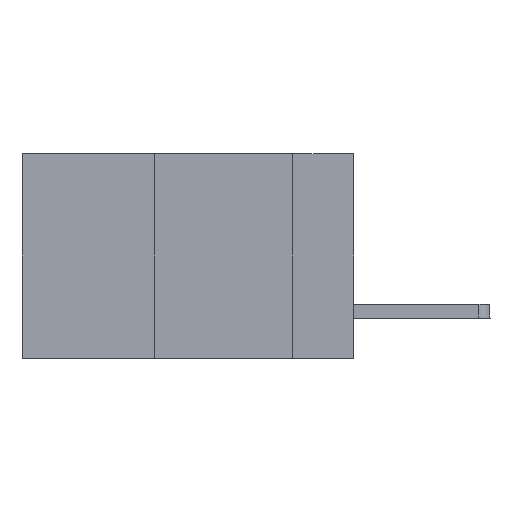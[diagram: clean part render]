
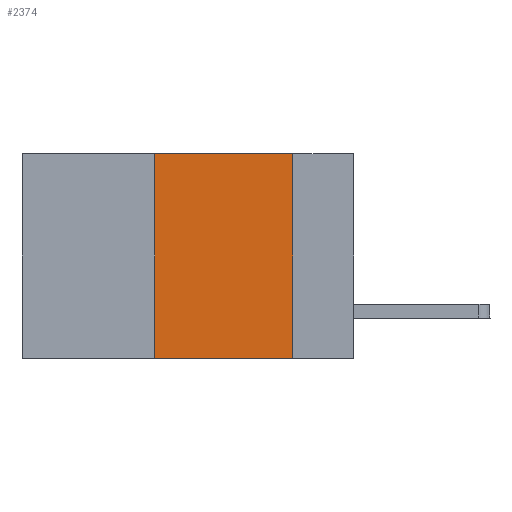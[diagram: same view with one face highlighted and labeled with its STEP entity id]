
A CAD part, left-side view. The second image highlights one B-rep face of the part: STEP entity #2374.
In plain terms, the highlighted planar face has unit normal (-1, 0, 0).
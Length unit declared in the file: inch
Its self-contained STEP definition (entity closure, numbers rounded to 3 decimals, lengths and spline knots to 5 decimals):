
#46 = EDGE_CURVE ( 'NONE', #2025, #4561, #7587, .T. ) ;
#168 = LINE ( 'NONE', #4430, #11557 ) ;
#1064 = VERTEX_POINT ( 'NONE', #3445 ) ;
#1229 = VERTEX_POINT ( 'NONE', #8865 ) ;
#1860 = CARTESIAN_POINT ( 'NONE',  ( 0., 0.11, 0. ) ) ;
#2025 = VERTEX_POINT ( 'NONE', #5776 ) ;
#2374 = ADVANCED_FACE ( 'NONE', ( #10381 ), #6928, .F. ) ;
#2579 = ORIENTED_EDGE ( 'NONE', *, *, #8840, .F. ) ;
#2673 = VECTOR ( 'NONE', #3794, 39.37008 ) ;
#2675 = VECTOR ( 'NONE', #6102, 39.37008 ) ;
#3445 = CARTESIAN_POINT ( 'NONE',  ( 0., 0.11, -0.37 ) ) ;
#3711 = EDGE_CURVE ( 'NONE', #1229, #2025, #168, .T. ) ;
#3794 = DIRECTION ( 'NONE',  ( 0., 0., -1. ) ) ;
#4235 = DIRECTION ( 'NONE',  ( 0., 0., -1. ) ) ;
#4430 = CARTESIAN_POINT ( 'NONE',  ( 0., 0.36, 0. ) ) ;
#4561 = VERTEX_POINT ( 'NONE', #9695 ) ;
#5181 = LINE ( 'NONE', #1860, #2673 ) ;
#5776 = CARTESIAN_POINT ( 'NONE',  ( 0., 0.36, 0. ) ) ;
#6102 = DIRECTION ( 'NONE',  ( 0., -1., 0. ) ) ;
#6368 = DIRECTION ( 'NONE',  ( 0., 0., 1. ) ) ;
#6550 = DIRECTION ( 'NONE',  ( 0., -1., 0. ) ) ;
#6928 = PLANE ( 'NONE',  #7059 ) ;
#7059 = AXIS2_PLACEMENT_3D ( 'NONE', #9151, #8613, #4235 ) ;
#7584 = VECTOR ( 'NONE', #6550, 39.37008 ) ;
#7587 = LINE ( 'NONE', #11451, #2675 ) ;
#8382 = ORIENTED_EDGE ( 'NONE', *, *, #46, .F. ) ;
#8613 = DIRECTION ( 'NONE',  ( 1., 0., 0. ) ) ;
#8840 = EDGE_CURVE ( 'NONE', #4561, #1064, #5181, .T. ) ;
#8855 = EDGE_CURVE ( 'NONE', #1229, #1064, #10034, .T. ) ;
#8865 = CARTESIAN_POINT ( 'NONE',  ( 0., 0.36, -0.37 ) ) ;
#8937 = ORIENTED_EDGE ( 'NONE', *, *, #3711, .F. ) ;
#9151 = CARTESIAN_POINT ( 'NONE',  ( 0., 0.6, 0. ) ) ;
#9695 = CARTESIAN_POINT ( 'NONE',  ( 0., 0.11, 0. ) ) ;
#10034 = LINE ( 'NONE', #10169, #7584 ) ;
#10169 = CARTESIAN_POINT ( 'NONE',  ( 0., 0.6, -0.37 ) ) ;
#10301 = EDGE_LOOP ( 'NONE', ( #2579, #8382, #8937, #11395 ) ) ;
#10381 = FACE_OUTER_BOUND ( 'NONE', #10301, .T. ) ;
#11395 = ORIENTED_EDGE ( 'NONE', *, *, #8855, .T. ) ;
#11451 = CARTESIAN_POINT ( 'NONE',  ( 0., 0.6, 0. ) ) ;
#11557 = VECTOR ( 'NONE', #6368, 39.37008 ) ;
